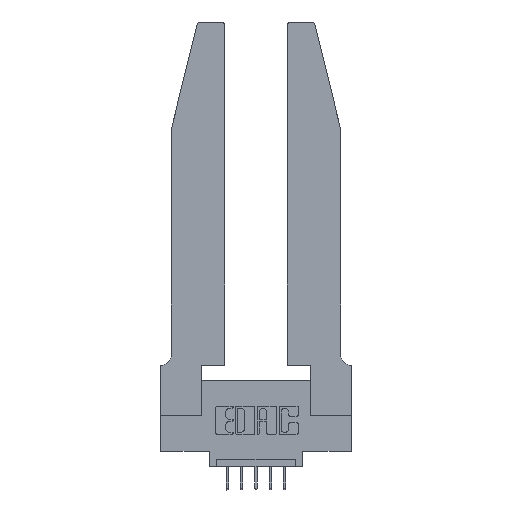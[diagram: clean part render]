
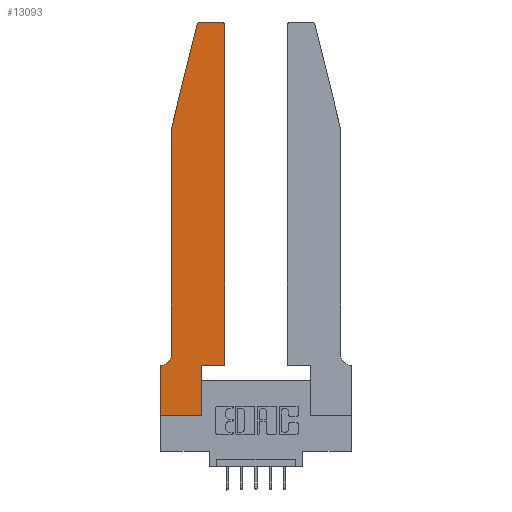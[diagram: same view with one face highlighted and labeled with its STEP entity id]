
A CAD part, top view. The second image highlights one B-rep face of the part: STEP entity #13093.
In plain terms, the highlighted planar face has unit normal (0, 0, 1).
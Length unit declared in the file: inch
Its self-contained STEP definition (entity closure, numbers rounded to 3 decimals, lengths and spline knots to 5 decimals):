
#368 = CARTESIAN_POINT ( 'NONE',  ( 0.4505, 2.72, 0.37 ) ) ;
#460 = ORIENTED_EDGE ( 'NONE', *, *, #12689, .T. ) ;
#560 = DIRECTION ( 'NONE',  ( -0.239, -0.971, 0. ) ) ;
#724 = PLANE ( 'NONE',  #1209 ) ;
#757 = DIRECTION ( 'NONE',  ( 0., 1., 0. ) ) ;
#764 = CIRCLE ( 'NONE', #6528, 0.07 ) ;
#1026 = DIRECTION ( 'NONE',  ( 1., 0., 0. ) ) ;
#1157 = DIRECTION ( 'NONE',  ( 1., 0., 0. ) ) ;
#1209 = AXIS2_PLACEMENT_3D ( 'NONE', #9189, #1651, #8155 ) ;
#1253 = CARTESIAN_POINT ( 'NONE',  ( 0.2865, 0.35, 0.37 ) ) ;
#1291 = LINE ( 'NONE', #12653, #1957 ) ;
#1602 = LINE ( 'NONE', #11482, #7582 ) ;
#1620 = VERTEX_POINT ( 'NONE', #10586 ) ;
#1651 = DIRECTION ( 'NONE',  ( 0., 0., 1. ) ) ;
#1796 = CARTESIAN_POINT ( 'NONE',  ( 0.0755, 2., 0.37 ) ) ;
#1914 = ORIENTED_EDGE ( 'NONE', *, *, #12350, .T. ) ;
#1957 = VECTOR ( 'NONE', #1026, 39.37008 ) ;
#2024 = CARTESIAN_POINT ( 'NONE',  ( 0.25487, 2.72718, 0.37 ) ) ;
#2272 = DIRECTION ( 'NONE',  ( -1., 0., 0. ) ) ;
#2321 = DIRECTION ( 'NONE',  ( 1., 0., 0. ) ) ;
#2398 = EDGE_CURVE ( 'NONE', #11092, #12570, #9006, .T. ) ;
#2417 = CARTESIAN_POINT ( 'NONE',  ( 0.4205, 2.75, 0.37 ) ) ;
#2765 = CARTESIAN_POINT ( 'NONE',  ( 0.0755, 2., 0.37 ) ) ;
#2868 = EDGE_LOOP ( 'NONE', ( #5860, #4596, #10215, #3412, #11932, #7537, #12499, #6344, #3173, #1914, #11100, #460 ) ) ;
#3002 = VERTEX_POINT ( 'NONE', #5185 ) ;
#3173 = ORIENTED_EDGE ( 'NONE', *, *, #4205, .T. ) ;
#3281 = CARTESIAN_POINT ( 'NONE',  ( 0.2605, 2.75, 0.37 ) ) ;
#3370 = LINE ( 'NONE', #3666, #5526 ) ;
#3412 = ORIENTED_EDGE ( 'NONE', *, *, #10149, .T. ) ;
#3639 = AXIS2_PLACEMENT_3D ( 'NONE', #13701, #11656, #1157 ) ;
#3666 = CARTESIAN_POINT ( 'NONE',  ( 0.2865, 0.35, 0.37 ) ) ;
#3782 = LINE ( 'NONE', #12966, #8909 ) ;
#4205 = EDGE_CURVE ( 'NONE', #10274, #9150, #3370, .T. ) ;
#4569 = CARTESIAN_POINT ( 'NONE',  ( 0.284, 2.72, 0.37 ) ) ;
#4596 = ORIENTED_EDGE ( 'NONE', *, *, #7418, .T. ) ;
#4614 = DIRECTION ( 'NONE',  ( 0., 0., 1. ) ) ;
#4701 = CARTESIAN_POINT ( 'NONE',  ( 0.0755, 2., 0.37 ) ) ;
#4762 = CARTESIAN_POINT ( 'NONE',  ( 0.4505, 0.35, 0.37 ) ) ;
#4819 = CARTESIAN_POINT ( 'NONE',  ( 0.2865, 0., 0.37 ) ) ;
#4886 = DIRECTION ( 'NONE',  ( -1., 0., 0. ) ) ;
#4904 = VECTOR ( 'NONE', #4886, 39.37008 ) ;
#5076 = LINE ( 'NONE', #4762, #12844 ) ;
#5185 = CARTESIAN_POINT ( 'NONE',  ( 0., 0.35, 0.37 ) ) ;
#5260 = VERTEX_POINT ( 'NONE', #5685 ) ;
#5290 = CARTESIAN_POINT ( 'NONE',  ( 0.4505, 0.35, 0.37 ) ) ;
#5526 = VECTOR ( 'NONE', #8799, 39.37008 ) ;
#5531 = VECTOR ( 'NONE', #560, 39.37008 ) ;
#5685 = CARTESIAN_POINT ( 'NONE',  ( 0.0055, 0.35, 0.37 ) ) ;
#5860 = ORIENTED_EDGE ( 'NONE', *, *, #6144, .T. ) ;
#6072 = EDGE_CURVE ( 'NONE', #1620, #10274, #1291, .T. ) ;
#6144 = EDGE_CURVE ( 'NONE', #9055, #7197, #9447, .T. ) ;
#6344 = ORIENTED_EDGE ( 'NONE', *, *, #6072, .T. ) ;
#6528 = AXIS2_PLACEMENT_3D ( 'NONE', #7321, #13592, #11640 ) ;
#6623 = VECTOR ( 'NONE', #2272, 39.37008 ) ;
#7048 = CIRCLE ( 'NONE', #3639, 0.03 ) ;
#7153 = CARTESIAN_POINT ( 'NONE',  ( 0.0755, 0.42, 0.37 ) ) ;
#7197 = VERTEX_POINT ( 'NONE', #8189 ) ;
#7219 = EDGE_CURVE ( 'NONE', #13369, #11305, #1602, .T. ) ;
#7321 = CARTESIAN_POINT ( 'NONE',  ( 0.0055, 0.42, 0.37 ) ) ;
#7418 = EDGE_CURVE ( 'NONE', #7197, #11092, #13521, .T. ) ;
#7440 = EDGE_CURVE ( 'NONE', #3002, #1620, #3782, .T. ) ;
#7537 = ORIENTED_EDGE ( 'NONE', *, *, #12425, .T. ) ;
#7582 = VECTOR ( 'NONE', #757, 39.37008 ) ;
#7908 = DIRECTION ( 'NONE',  ( 1., 0., 0. ) ) ;
#8155 = DIRECTION ( 'NONE',  ( 1., 0., 0. ) ) ;
#8189 = CARTESIAN_POINT ( 'NONE',  ( 0.284, 2.75, 0.37 ) ) ;
#8799 = DIRECTION ( 'NONE',  ( 0., 1., 0. ) ) ;
#8909 = VECTOR ( 'NONE', #9854, 39.37008 ) ;
#9006 = LINE ( 'NONE', #4701, #5531 ) ;
#9055 = VERTEX_POINT ( 'NONE', #2417 ) ;
#9114 = CARTESIAN_POINT ( 'NONE',  ( 0.0755, 0.35, 0.37 ) ) ;
#9150 = VERTEX_POINT ( 'NONE', #1253 ) ;
#9189 = CARTESIAN_POINT ( 'NONE',  ( 0., 0.35, 0.37 ) ) ;
#9447 = LINE ( 'NONE', #3281, #6623 ) ;
#9854 = DIRECTION ( 'NONE',  ( 0., -1., 0. ) ) ;
#9924 = EDGE_CURVE ( 'NONE', #12647, #5260, #764, .T. ) ;
#10149 = EDGE_CURVE ( 'NONE', #12570, #12647, #11774, .T. ) ;
#10215 = ORIENTED_EDGE ( 'NONE', *, *, #2398, .T. ) ;
#10274 = VERTEX_POINT ( 'NONE', #4819 ) ;
#10586 = CARTESIAN_POINT ( 'NONE',  ( 0., 0., 0.37 ) ) ;
#11092 = VERTEX_POINT ( 'NONE', #2024 ) ;
#11100 = ORIENTED_EDGE ( 'NONE', *, *, #7219, .T. ) ;
#11212 = LINE ( 'NONE', #9114, #4904 ) ;
#11305 = VERTEX_POINT ( 'NONE', #368 ) ;
#11482 = CARTESIAN_POINT ( 'NONE',  ( 0.4505, 0.35, 0.37 ) ) ;
#11640 = DIRECTION ( 'NONE',  ( -1., 0., 0. ) ) ;
#11656 = DIRECTION ( 'NONE',  ( 0., 0., 1. ) ) ;
#11774 = LINE ( 'NONE', #2765, #12099 ) ;
#11932 = ORIENTED_EDGE ( 'NONE', *, *, #9924, .T. ) ;
#12099 = VECTOR ( 'NONE', #13394, 39.37008 ) ;
#12349 = AXIS2_PLACEMENT_3D ( 'NONE', #4569, #4614, #2321 ) ;
#12350 = EDGE_CURVE ( 'NONE', #9150, #13369, #5076, .T. ) ;
#12425 = EDGE_CURVE ( 'NONE', #5260, #3002, #11212, .T. ) ;
#12499 = ORIENTED_EDGE ( 'NONE', *, *, #7440, .T. ) ;
#12570 = VERTEX_POINT ( 'NONE', #1796 ) ;
#12647 = VERTEX_POINT ( 'NONE', #7153 ) ;
#12653 = CARTESIAN_POINT ( 'NONE',  ( 0., 0., 0.37 ) ) ;
#12689 = EDGE_CURVE ( 'NONE', #11305, #9055, #7048, .T. ) ;
#12844 = VECTOR ( 'NONE', #7908, 39.37008 ) ;
#12966 = CARTESIAN_POINT ( 'NONE',  ( 0., 0., 0.37 ) ) ;
#13093 = ADVANCED_FACE ( 'NONE', ( #13135 ), #724, .T. ) ;
#13135 = FACE_OUTER_BOUND ( 'NONE', #2868, .T. ) ;
#13369 = VERTEX_POINT ( 'NONE', #5290 ) ;
#13394 = DIRECTION ( 'NONE',  ( 0., -1., 0. ) ) ;
#13521 = CIRCLE ( 'NONE', #12349, 0.03 ) ;
#13592 = DIRECTION ( 'NONE',  ( 0., 0., -1. ) ) ;
#13701 = CARTESIAN_POINT ( 'NONE',  ( 0.4205, 2.72, 0.37 ) ) ;
